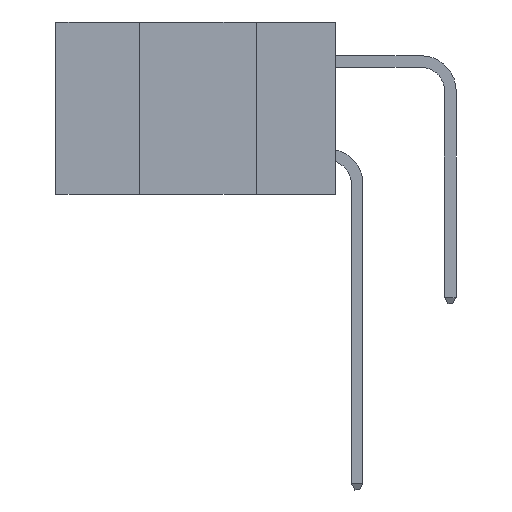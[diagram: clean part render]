
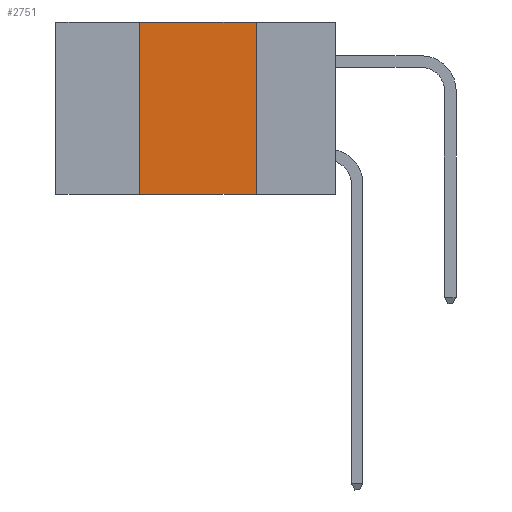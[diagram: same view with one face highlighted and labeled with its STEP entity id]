
A CAD part, left-side view. The second image highlights one B-rep face of the part: STEP entity #2751.
In plain terms, the highlighted planar face has unit normal (-1, 0, 0).
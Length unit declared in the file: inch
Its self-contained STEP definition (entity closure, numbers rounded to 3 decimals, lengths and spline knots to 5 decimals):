
#41 = VECTOR ( 'NONE', #9846, 39.37008 ) ;
#2122 = EDGE_CURVE ( 'NONE', #3568, #9568, #2442, .T. ) ;
#2377 = DIRECTION ( 'NONE',  ( 0., 0., -1. ) ) ;
#2442 = LINE ( 'NONE', #5406, #4758 ) ;
#2751 = ADVANCED_FACE ( 'NONE', ( #16350 ), #17939, .F. ) ;
#3071 = ORIENTED_EDGE ( 'NONE', *, *, #8012, .F. ) ;
#3568 = VERTEX_POINT ( 'NONE', #5475 ) ;
#3695 = CARTESIAN_POINT ( 'NONE',  ( 0., 0.6, 0. ) ) ;
#4758 = VECTOR ( 'NONE', #17987, 39.37008 ) ;
#5406 = CARTESIAN_POINT ( 'NONE',  ( 0., 0.42, 0. ) ) ;
#5475 = CARTESIAN_POINT ( 'NONE',  ( 0., 0.42, -0.37 ) ) ;
#5699 = VECTOR ( 'NONE', #6907, 39.37008 ) ;
#5930 = CARTESIAN_POINT ( 'NONE',  ( 0., 0.6, 0. ) ) ;
#6363 = ORIENTED_EDGE ( 'NONE', *, *, #9771, .T. ) ;
#6519 = CARTESIAN_POINT ( 'NONE',  ( 0., 0.42, 0. ) ) ;
#6907 = DIRECTION ( 'NONE',  ( 0., 0., -1. ) ) ;
#7792 = VERTEX_POINT ( 'NONE', #15038 ) ;
#8012 = EDGE_CURVE ( 'NONE', #8906, #7792, #12286, .T. ) ;
#8906 = VERTEX_POINT ( 'NONE', #18220 ) ;
#9482 = ORIENTED_EDGE ( 'NONE', *, *, #18239, .F. ) ;
#9568 = VERTEX_POINT ( 'NONE', #6519 ) ;
#9771 = EDGE_CURVE ( 'NONE', #3568, #7792, #17990, .T. ) ;
#9846 = DIRECTION ( 'NONE',  ( 0., -1., 0. ) ) ;
#11567 = DIRECTION ( 'NONE',  ( 0., -1., 0. ) ) ;
#12286 = LINE ( 'NONE', #18095, #5699 ) ;
#12960 = LINE ( 'NONE', #5930, #16407 ) ;
#15038 = CARTESIAN_POINT ( 'NONE',  ( 0., 0.17, -0.37 ) ) ;
#15048 = DIRECTION ( 'NONE',  ( 1., 0., 0. ) ) ;
#15352 = ORIENTED_EDGE ( 'NONE', *, *, #2122, .F. ) ;
#15467 = AXIS2_PLACEMENT_3D ( 'NONE', #3695, #15048, #2377 ) ;
#16350 = FACE_OUTER_BOUND ( 'NONE', #17132, .T. ) ;
#16407 = VECTOR ( 'NONE', #11567, 39.37008 ) ;
#17132 = EDGE_LOOP ( 'NONE', ( #3071, #9482, #15352, #6363 ) ) ;
#17939 = PLANE ( 'NONE',  #15467 ) ;
#17987 = DIRECTION ( 'NONE',  ( 0., 0., 1. ) ) ;
#17990 = LINE ( 'NONE', #18265, #41 ) ;
#18095 = CARTESIAN_POINT ( 'NONE',  ( 0., 0.17, 0. ) ) ;
#18220 = CARTESIAN_POINT ( 'NONE',  ( 0., 0.17, 0. ) ) ;
#18239 = EDGE_CURVE ( 'NONE', #9568, #8906, #12960, .T. ) ;
#18265 = CARTESIAN_POINT ( 'NONE',  ( 0., 0.6, -0.37 ) ) ;
